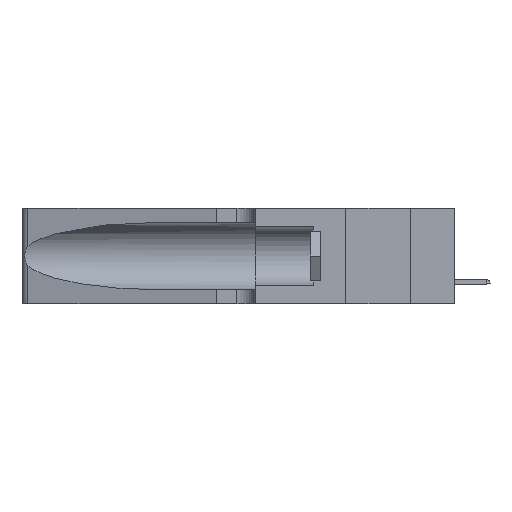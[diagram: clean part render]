
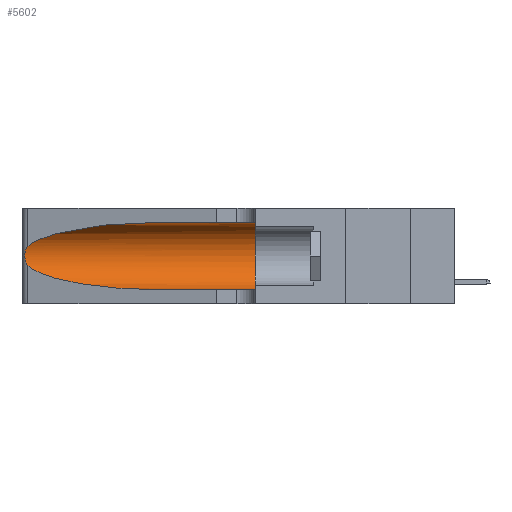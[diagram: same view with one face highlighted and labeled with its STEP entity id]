
A CAD part, left-side view. The second image highlights one B-rep face of the part: STEP entity #5602.
In plain terms, the highlighted cylindrical face has radius 3.308 mm (diameter 6.617 mm), a partial arc.
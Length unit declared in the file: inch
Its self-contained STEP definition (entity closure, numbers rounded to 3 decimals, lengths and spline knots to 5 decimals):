
#549 = EDGE_CURVE ( 'NONE', #27941, #23967, #3049, .T. ) ;
#598 = CARTESIAN_POINT ( 'NONE',  ( 0.26075, 1.23896, 0.19203 ) ) ;
#1314 = AXIS2_PLACEMENT_3D ( 'NONE', #19859, #7649, #29966 ) ;
#1413 = VECTOR ( 'NONE', #27132, 39.37008 ) ;
#3010 = CARTESIAN_POINT ( 'NONE',  ( 0.25639, 1.23184, 0.21858 ) ) ;
#3049 = B_SPLINE_CURVE_WITH_KNOTS ( 'NONE', 3,
 ( #27883, #7864, #3010, #8499, #18083, #17763, #598, #6051, #5578, #15935, #18418, #27730, #30641, #8335 ),
 .UNSPECIFIED., .F., .F.,
 ( 4, 2, 2, 2, 2, 2, 4 ),
 ( 0., 0.00027, 0.00053, 0.00107, 0.0016, 0.00187, 0.00214 ),
 .UNSPECIFIED. ) ;
#4995 = LINE ( 'NONE', #9682, #1413 ) ;
#5313 =( BOUNDED_CURVE ( )  B_SPLINE_CURVE ( 3, ( #7883, #12892, #20413, #10472 ),
 .UNSPECIFIED., .F., .T. ) 
 B_SPLINE_CURVE_WITH_KNOTS ( ( 4, 4 ),
 ( 1.5708, 2.84003 ),
 .UNSPECIFIED. ) 
 CURVE ( )  GEOMETRIC_REPRESENTATION_ITEM ( )  RATIONAL_B_SPLINE_CURVE ( ( 1., 0.87, 0.87, 1. ) ) 
 REPRESENTATION_ITEM ( '' )  );
#5578 = CARTESIAN_POINT ( 'NONE',  ( 0.26017, 1.23833, 0.17102 ) ) ;
#5602 = ADVANCED_FACE ( 'NONE', ( #14186 ), #13855, .F. ) ;
#5838 = EDGE_CURVE ( 'NONE', #31175, #5938, #4995, .T. ) ;
#5938 = VERTEX_POINT ( 'NONE', #20443 ) ;
#6008 = CARTESIAN_POINT ( 'NONE',  ( 0.1305, 0.72297, 0.05475 ) ) ;
#6051 = CARTESIAN_POINT ( 'NONE',  ( 0.26075, 1.23896, 0.178 ) ) ;
#6052 = ORIENTED_EDGE ( 'NONE', *, *, #18604, .T. ) ;
#6147 = CARTESIAN_POINT ( 'NONE',  ( 0.25487, 1.22718, 0.14631 ) ) ;
#7552 = CIRCLE ( 'NONE', #1314, 0.13025 ) ;
#7649 = DIRECTION ( 'NONE',  ( 0., 1., 0. ) ) ;
#7864 = CARTESIAN_POINT ( 'NONE',  ( 0.25555, 1.22994, 0.2215 ) ) ;
#7883 = CARTESIAN_POINT ( 'NONE',  ( 0.1305, 0.72297, 0.31525 ) ) ;
#8335 = CARTESIAN_POINT ( 'NONE',  ( 0.25487, 1.22718, 0.14631 ) ) ;
#8499 = CARTESIAN_POINT ( 'NONE',  ( 0.25787, 1.23484, 0.2124 ) ) ;
#8859 = DIRECTION ( 'NONE',  ( 0., -1., 0. ) ) ;
#9682 = CARTESIAN_POINT ( 'NONE',  ( 0.1305, 1.61858, 0.31525 ) ) ;
#10031 =( BOUNDED_CURVE ( )  B_SPLINE_CURVE ( 3, ( #6147, #26331, #16029, #26025 ),
 .UNSPECIFIED., .F., .T. ) 
 B_SPLINE_CURVE_WITH_KNOTS ( ( 4, 4 ),
 ( 3.44316, 4.71239 ),
 .UNSPECIFIED. ) 
 CURVE ( )  GEOMETRIC_REPRESENTATION_ITEM ( )  RATIONAL_B_SPLINE_CURVE ( ( 1., 0.87, 0.87, 1. ) ) 
 REPRESENTATION_ITEM ( '' )  );
#10472 = CARTESIAN_POINT ( 'NONE',  ( 0.25487, 1.22718, 0.22369 ) ) ;
#11288 = LINE ( 'NONE', #13722, #18994 ) ;
#12892 = CARTESIAN_POINT ( 'NONE',  ( 0.18966, 0.96281, 0.31525 ) ) ;
#13722 = CARTESIAN_POINT ( 'NONE',  ( 0.1305, 1.61858, 0.05475 ) ) ;
#13855 = CYLINDRICAL_SURFACE ( 'NONE', #27131, 0.13025 ) ;
#14186 = FACE_OUTER_BOUND ( 'NONE', #17447, .T. ) ;
#15175 = EDGE_CURVE ( 'NONE', #5938, #29880, #7552, .T. ) ;
#15377 = VERTEX_POINT ( 'NONE', #6008 ) ;
#15935 = CARTESIAN_POINT ( 'NONE',  ( 0.25856, 1.23593, 0.16098 ) ) ;
#16029 = CARTESIAN_POINT ( 'NONE',  ( 0.18966, 0.96281, 0.05475 ) ) ;
#17447 = EDGE_LOOP ( 'NONE', ( #6052, #20950, #22481, #23139, #25335, #31181 ) ) ;
#17763 = CARTESIAN_POINT ( 'NONE',  ( 0.26018, 1.23835, 0.19895 ) ) ;
#18083 = CARTESIAN_POINT ( 'NONE',  ( 0.25854, 1.2359, 0.20912 ) ) ;
#18418 = CARTESIAN_POINT ( 'NONE',  ( 0.25789, 1.23486, 0.15765 ) ) ;
#18477 = DIRECTION ( 'NONE',  ( 0., -1., 0. ) ) ;
#18604 = EDGE_CURVE ( 'NONE', #31175, #27941, #5313, .T. ) ;
#18994 = VECTOR ( 'NONE', #18477, 39.37008 ) ;
#19257 = CARTESIAN_POINT ( 'NONE',  ( 0.1305, 1.61858, 0.185 ) ) ;
#19643 = EDGE_CURVE ( 'NONE', #23967, #15377, #10031, .T. ) ;
#19754 = CARTESIAN_POINT ( 'NONE',  ( 0.25487, 1.22718, 0.14631 ) ) ;
#19841 = EDGE_CURVE ( 'NONE', #15377, #29880, #11288, .T. ) ;
#19859 = CARTESIAN_POINT ( 'NONE',  ( 0.1305, 0.35, 0.185 ) ) ;
#20413 = CARTESIAN_POINT ( 'NONE',  ( 0.2373, 1.15595, 0.28018 ) ) ;
#20443 = CARTESIAN_POINT ( 'NONE',  ( 0.1305, 0.35, 0.31525 ) ) ;
#20950 = ORIENTED_EDGE ( 'NONE', *, *, #549, .T. ) ;
#22481 = ORIENTED_EDGE ( 'NONE', *, *, #19643, .T. ) ;
#23139 = ORIENTED_EDGE ( 'NONE', *, *, #19841, .T. ) ;
#23967 = VERTEX_POINT ( 'NONE', #19754 ) ;
#25011 = CARTESIAN_POINT ( 'NONE',  ( 0.25487, 1.22718, 0.22369 ) ) ;
#25335 = ORIENTED_EDGE ( 'NONE', *, *, #15175, .F. ) ;
#26025 = CARTESIAN_POINT ( 'NONE',  ( 0.1305, 0.72297, 0.05475 ) ) ;
#26331 = CARTESIAN_POINT ( 'NONE',  ( 0.2373, 1.15595, 0.08982 ) ) ;
#27131 = AXIS2_PLACEMENT_3D ( 'NONE', #19257, #8859, #31477 ) ;
#27132 = DIRECTION ( 'NONE',  ( 0., -1., 0. ) ) ;
#27730 = CARTESIAN_POINT ( 'NONE',  ( 0.25639, 1.23186, 0.15144 ) ) ;
#27883 = CARTESIAN_POINT ( 'NONE',  ( 0.25487, 1.22718, 0.22369 ) ) ;
#27941 = VERTEX_POINT ( 'NONE', #25011 ) ;
#29432 = CARTESIAN_POINT ( 'NONE',  ( 0.1305, 0.72297, 0.31525 ) ) ;
#29880 = VERTEX_POINT ( 'NONE', #31577 ) ;
#29966 = DIRECTION ( 'NONE',  ( 0., 0., 1. ) ) ;
#30641 = CARTESIAN_POINT ( 'NONE',  ( 0.25555, 1.22993, 0.14849 ) ) ;
#31175 = VERTEX_POINT ( 'NONE', #29432 ) ;
#31181 = ORIENTED_EDGE ( 'NONE', *, *, #5838, .F. ) ;
#31477 = DIRECTION ( 'NONE',  ( 0., 0., -1. ) ) ;
#31577 = CARTESIAN_POINT ( 'NONE',  ( 0.1305, 0.35, 0.05475 ) ) ;
